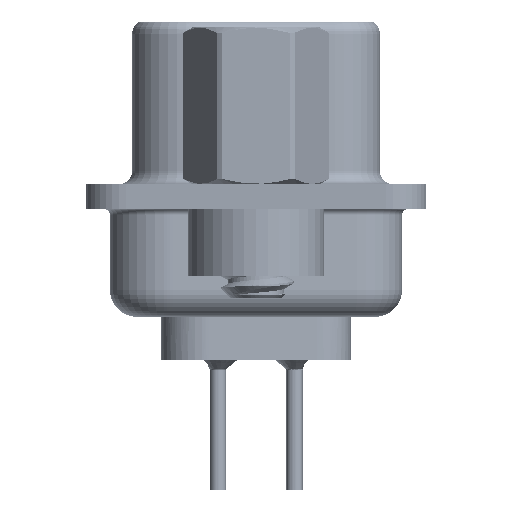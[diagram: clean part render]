
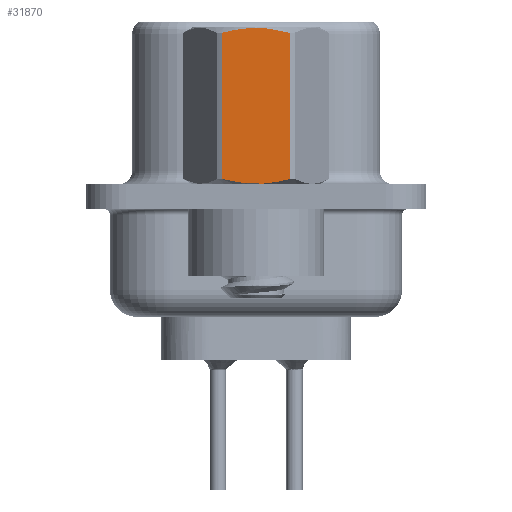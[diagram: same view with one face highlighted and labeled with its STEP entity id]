
A CAD part, left-side view. The second image highlights one B-rep face of the part: STEP entity #31870.
In plain terms, the highlighted planar face has unit normal (-1, 0, 0).
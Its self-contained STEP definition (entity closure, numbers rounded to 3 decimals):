
#481 = AXIS2_PLACEMENT_3D ( 'NONE', #16404, #12396, #9797 ) ;
#1683 = CARTESIAN_POINT ( 'NONE',  ( -2.381, 0.853, 0.549 ) ) ;
#1844 = PLANE ( 'NONE',  #481 ) ;
#1937 = LINE ( 'NONE', #15752, #30908 ) ;
#2748 = VERTEX_POINT ( 'NONE', #23654 ) ;
#2822 = CARTESIAN_POINT ( 'NONE',  ( -2.381, 1.273, 0.652 ) ) ;
#3050 = VERTEX_POINT ( 'NONE', #27798 ) ;
#3190 = B_SPLINE_CURVE_WITH_KNOTS ( 'NONE', 3,
 ( #6244, #27380, #25141, #24964, #19926, #14029, #11956, #16805, #19580, #30317 ),
 .UNSPECIFIED., .F., .F.,
 ( 4, 2, 2, 2, 4 ),
 ( 0.001, 0.002, 0.002, 0.003, 0.004 ),
 .UNSPECIFIED. ) ;
#3238 = EDGE_LOOP ( 'NONE', ( #4420, #25870, #9342, #5531 ) ) ;
#4100 = CARTESIAN_POINT ( 'NONE',  ( -2.381, -0.432, 0.485 ) ) ;
#4420 = ORIENTED_EDGE ( 'NONE', *, *, #20505, .T. ) ;
#5531 = ORIENTED_EDGE ( 'NONE', *, *, #33553, .T. ) ;
#6244 = CARTESIAN_POINT ( 'NONE',  ( -2.381, -1.273, 6.048 ) ) ;
#8472 = CARTESIAN_POINT ( 'NONE',  ( -2.381, -1.273, 3.792 ) ) ;
#9129 = CARTESIAN_POINT ( 'NONE',  ( -2.381, -1.273, 0.652 ) ) ;
#9342 = ORIENTED_EDGE ( 'NONE', *, *, #27549, .T. ) ;
#9797 = DIRECTION ( 'NONE',  ( 0., -1., 0. ) ) ;
#9977 = CARTESIAN_POINT ( 'NONE',  ( -2.381, 1.273, 0.652 ) ) ;
#11838 = VERTEX_POINT ( 'NONE', #2822 ) ;
#11956 = CARTESIAN_POINT ( 'NONE',  ( -2.381, 0.428, 6.215 ) ) ;
#12396 = DIRECTION ( 'NONE',  ( -1., 0., 0. ) ) ;
#13415 = VECTOR ( 'NONE', #16769, 1000. ) ;
#14029 = CARTESIAN_POINT ( 'NONE',  ( -2.381, 0.215, 6.232 ) ) ;
#14653 = CARTESIAN_POINT ( 'NONE',  ( -2.381, 0.428, 0.485 ) ) ;
#15752 = CARTESIAN_POINT ( 'NONE',  ( -2.381, 1.273, 3.792 ) ) ;
#15864 = EDGE_CURVE ( 'NONE', #17592, #2748, #24211, .T. ) ;
#16404 = CARTESIAN_POINT ( 'NONE',  ( -2.381, 1.375, -3.75 ) ) ;
#16769 = DIRECTION ( 'NONE',  ( 0., 0., 1. ) ) ;
#16805 = CARTESIAN_POINT ( 'NONE',  ( -2.381, 0.853, 6.151 ) ) ;
#17592 = VERTEX_POINT ( 'NONE', #9129 ) ;
#18018 = DIRECTION ( 'NONE',  ( 0., 0., -1. ) ) ;
#19580 = CARTESIAN_POINT ( 'NONE',  ( -2.381, 1.065, 6.104 ) ) ;
#19926 = CARTESIAN_POINT ( 'NONE',  ( -2.381, -0.215, 6.232 ) ) ;
#20505 = EDGE_CURVE ( 'NONE', #11838, #17592, #24293, .T. ) ;
#23654 = CARTESIAN_POINT ( 'NONE',  ( -2.381, -1.273, 6.048 ) ) ;
#24211 = LINE ( 'NONE', #8472, #13415 ) ;
#24293 = B_SPLINE_CURVE_WITH_KNOTS ( 'NONE', 3,
 ( #9977, #30425, #1683, #14653, #27825, #30248, #4100, #33705, #30594, #25231 ),
 .UNSPECIFIED., .F., .F.,
 ( 4, 2, 2, 2, 4 ),
 ( 0.003, 0.003, 0.004, 0.004, 0.005 ),
 .UNSPECIFIED. ) ;
#24964 = CARTESIAN_POINT ( 'NONE',  ( -2.381, -0.432, 6.215 ) ) ;
#25141 = CARTESIAN_POINT ( 'NONE',  ( -2.381, -0.858, 6.15 ) ) ;
#25231 = CARTESIAN_POINT ( 'NONE',  ( -2.381, -1.273, 0.652 ) ) ;
#25562 = FACE_OUTER_BOUND ( 'NONE', #3238, .T. ) ;
#25870 = ORIENTED_EDGE ( 'NONE', *, *, #15864, .T. ) ;
#27380 = CARTESIAN_POINT ( 'NONE',  ( -2.381, -1.066, 6.104 ) ) ;
#27549 = EDGE_CURVE ( 'NONE', #2748, #3050, #3190, .T. ) ;
#27798 = CARTESIAN_POINT ( 'NONE',  ( -2.381, 1.273, 6.048 ) ) ;
#27825 = CARTESIAN_POINT ( 'NONE',  ( -2.381, 0.215, 0.468 ) ) ;
#30248 = CARTESIAN_POINT ( 'NONE',  ( -2.381, -0.215, 0.468 ) ) ;
#30317 = CARTESIAN_POINT ( 'NONE',  ( -2.381, 1.273, 6.048 ) ) ;
#30425 = CARTESIAN_POINT ( 'NONE',  ( -2.381, 1.065, 0.596 ) ) ;
#30594 = CARTESIAN_POINT ( 'NONE',  ( -2.381, -1.066, 0.596 ) ) ;
#30908 = VECTOR ( 'NONE', #18018, 1000. ) ;
#31870 = ADVANCED_FACE ( 'NONE', ( #25562 ), #1844, .T. ) ;
#33553 = EDGE_CURVE ( 'NONE', #3050, #11838, #1937, .T. ) ;
#33705 = CARTESIAN_POINT ( 'NONE',  ( -2.381, -0.858, 0.55 ) ) ;
